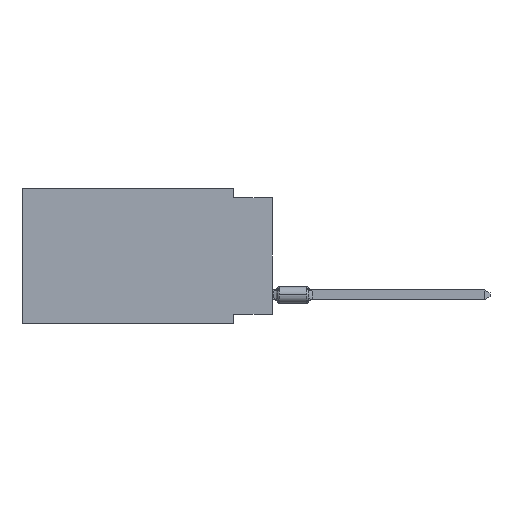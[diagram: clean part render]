
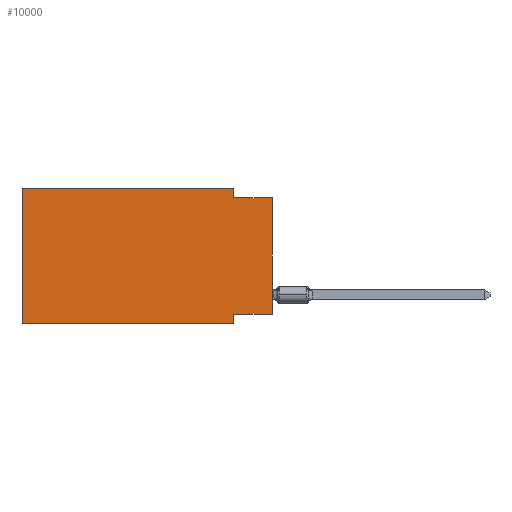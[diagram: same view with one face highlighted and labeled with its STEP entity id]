
A CAD part, left-side view. The second image highlights one B-rep face of the part: STEP entity #10000.
In plain terms, the highlighted planar face has unit normal (-1, 0, 0).
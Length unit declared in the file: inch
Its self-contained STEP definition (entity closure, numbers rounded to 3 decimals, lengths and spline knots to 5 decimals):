
#117 = CARTESIAN_POINT ( 'NONE',  ( 0., 0.645, 0. ) ) ;
#170 = EDGE_CURVE ( 'NONE', #8030, #2057, #592, .T. ) ;
#196 = CARTESIAN_POINT ( 'NONE',  ( 0., 0.645, 0. ) ) ;
#272 = VERTEX_POINT ( 'NONE', #16526 ) ;
#276 = CARTESIAN_POINT ( 'NONE',  ( 0., 0., -0.025 ) ) ;
#592 = LINE ( 'NONE', #16163, #17662 ) ;
#788 = ORIENTED_EDGE ( 'NONE', *, *, #1704, .F. ) ;
#1298 = CARTESIAN_POINT ( 'NONE',  ( 0., 0.1, -0.35 ) ) ;
#1704 = EDGE_CURVE ( 'NONE', #13921, #4736, #11565, .T. ) ;
#2057 = VERTEX_POINT ( 'NONE', #276 ) ;
#2071 = CARTESIAN_POINT ( 'NONE',  ( 0., 0.1, -0.35 ) ) ;
#2440 = ORIENTED_EDGE ( 'NONE', *, *, #15924, .F. ) ;
#2850 = CARTESIAN_POINT ( 'NONE',  ( 0., 0.1, 0. ) ) ;
#2868 = CARTESIAN_POINT ( 'NONE',  ( 0., 0.645, 0. ) ) ;
#3587 = VERTEX_POINT ( 'NONE', #4905 ) ;
#3730 = EDGE_CURVE ( 'NONE', #8164, #3587, #4223, .T. ) ;
#3893 = LINE ( 'NONE', #5461, #13225 ) ;
#4066 = DIRECTION ( 'NONE',  ( 1., 0., 0. ) ) ;
#4150 = DIRECTION ( 'NONE',  ( 0., 0., -1. ) ) ;
#4223 = LINE ( 'NONE', #2850, #9430 ) ;
#4540 = DIRECTION ( 'NONE',  ( 0., 0., -1. ) ) ;
#4613 = CARTESIAN_POINT ( 'NONE',  ( 0., 0.645, -0.35 ) ) ;
#4633 = DIRECTION ( 'NONE',  ( 0., -1., 0. ) ) ;
#4710 = DIRECTION ( 'NONE',  ( 0., 0., 1. ) ) ;
#4736 = VERTEX_POINT ( 'NONE', #14147 ) ;
#4905 = CARTESIAN_POINT ( 'NONE',  ( 0., 0.1, -0.025 ) ) ;
#4968 = ORIENTED_EDGE ( 'NONE', *, *, #17248, .F. ) ;
#5283 = VERTEX_POINT ( 'NONE', #1298 ) ;
#5372 = CARTESIAN_POINT ( 'NONE',  ( 0., 0.645, -0.35 ) ) ;
#5398 = VECTOR ( 'NONE', #8625, 39.37008 ) ;
#5461 = CARTESIAN_POINT ( 'NONE',  ( 0., 0., -0.325 ) ) ;
#5562 = ORIENTED_EDGE ( 'NONE', *, *, #3730, .F. ) ;
#5604 = DIRECTION ( 'NONE',  ( 0., 0., -1. ) ) ;
#6446 = ORIENTED_EDGE ( 'NONE', *, *, #15973, .F. ) ;
#6825 = DIRECTION ( 'NONE',  ( 0., 1., 0. ) ) ;
#8030 = VERTEX_POINT ( 'NONE', #10972 ) ;
#8164 = VERTEX_POINT ( 'NONE', #15532 ) ;
#8268 = PLANE ( 'NONE',  #15692 ) ;
#8481 = EDGE_LOOP ( 'NONE', ( #11147, #6446, #5562, #8855, #788, #16048, #2440, #4968 ) ) ;
#8625 = DIRECTION ( 'NONE',  ( 0., 0., 1. ) ) ;
#8855 = ORIENTED_EDGE ( 'NONE', *, *, #11559, .F. ) ;
#9430 = VECTOR ( 'NONE', #5604, 39.37008 ) ;
#10000 = ADVANCED_FACE ( 'NONE', ( #12393 ), #8268, .F. ) ;
#10200 = DIRECTION ( 'NONE',  ( 0., -1., 0. ) ) ;
#10972 = CARTESIAN_POINT ( 'NONE',  ( 0., 0., -0.325 ) ) ;
#11147 = ORIENTED_EDGE ( 'NONE', *, *, #170, .T. ) ;
#11559 = EDGE_CURVE ( 'NONE', #4736, #8164, #14022, .T. ) ;
#11565 = LINE ( 'NONE', #117, #5398 ) ;
#11696 = VECTOR ( 'NONE', #4633, 39.37008 ) ;
#12393 = FACE_OUTER_BOUND ( 'NONE', #8481, .T. ) ;
#12457 = VECTOR ( 'NONE', #14372, 39.37008 ) ;
#13225 = VECTOR ( 'NONE', #6825, 39.37008 ) ;
#13921 = VERTEX_POINT ( 'NONE', #5372 ) ;
#14022 = LINE ( 'NONE', #196, #12457 ) ;
#14147 = CARTESIAN_POINT ( 'NONE',  ( 0., 0.645, 0. ) ) ;
#14372 = DIRECTION ( 'NONE',  ( 0., -1., 0. ) ) ;
#14417 = CARTESIAN_POINT ( 'NONE',  ( 0., 0., -0.025 ) ) ;
#15532 = CARTESIAN_POINT ( 'NONE',  ( 0., 0.1, 0. ) ) ;
#15692 = AXIS2_PLACEMENT_3D ( 'NONE', #2868, #4066, #4150 ) ;
#15793 = VECTOR ( 'NONE', #4540, 39.37008 ) ;
#15924 = EDGE_CURVE ( 'NONE', #272, #5283, #17367, .T. ) ;
#15973 = EDGE_CURVE ( 'NONE', #3587, #2057, #17096, .T. ) ;
#16048 = ORIENTED_EDGE ( 'NONE', *, *, #17592, .T. ) ;
#16163 = CARTESIAN_POINT ( 'NONE',  ( 0., 0., 0. ) ) ;
#16526 = CARTESIAN_POINT ( 'NONE',  ( 0., 0.1, -0.325 ) ) ;
#16759 = VECTOR ( 'NONE', #10200, 39.37008 ) ;
#17096 = LINE ( 'NONE', #14417, #11696 ) ;
#17163 = LINE ( 'NONE', #4613, #16759 ) ;
#17248 = EDGE_CURVE ( 'NONE', #8030, #272, #3893, .T. ) ;
#17367 = LINE ( 'NONE', #2071, #15793 ) ;
#17592 = EDGE_CURVE ( 'NONE', #13921, #5283, #17163, .T. ) ;
#17662 = VECTOR ( 'NONE', #4710, 39.37008 ) ;
